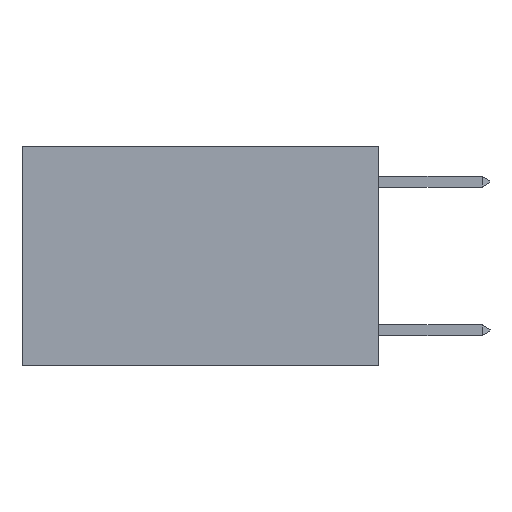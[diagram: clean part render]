
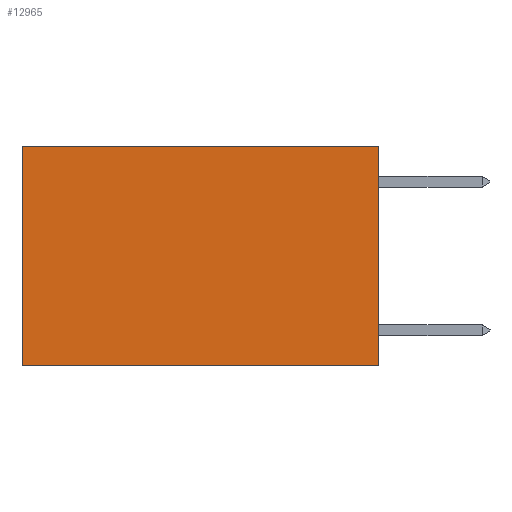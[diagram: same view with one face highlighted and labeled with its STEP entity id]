
A CAD part, left-side view. The second image highlights one B-rep face of the part: STEP entity #12965.
In plain terms, the highlighted planar face has unit normal (-1, 0, 0).
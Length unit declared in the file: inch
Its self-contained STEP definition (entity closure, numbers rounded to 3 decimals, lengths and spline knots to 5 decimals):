
#112 = VERTEX_POINT ( 'NONE', #4835 ) ;
#635 = DIRECTION ( 'NONE',  ( 0., 0., -1. ) ) ;
#2063 = FACE_OUTER_BOUND ( 'NONE', #7457, .T. ) ;
#2075 = EDGE_CURVE ( 'NONE', #17356, #7688, #20302, .T. ) ;
#2147 = EDGE_CURVE ( 'NONE', #112, #8916, #19720, .T. ) ;
#3076 = DIRECTION ( 'NONE',  ( 0., 1., 0. ) ) ;
#3376 = AXIS2_PLACEMENT_3D ( 'NONE', #9734, #11504, #635 ) ;
#4444 = EDGE_CURVE ( 'NONE', #8916, #7688, #9102, .T. ) ;
#4835 = CARTESIAN_POINT ( 'NONE',  ( 0.2625, 0., 0. ) ) ;
#5804 = CARTESIAN_POINT ( 'NONE',  ( 0.2625, 0.6, -0.37 ) ) ;
#7457 = EDGE_LOOP ( 'NONE', ( #9410, #13491, #9125, #22528 ) ) ;
#7688 = VERTEX_POINT ( 'NONE', #5804 ) ;
#8466 = CARTESIAN_POINT ( 'NONE',  ( 0.2625, 0., -0.37 ) ) ;
#8916 = VERTEX_POINT ( 'NONE', #8466 ) ;
#9102 = LINE ( 'NONE', #14715, #9173 ) ;
#9125 = ORIENTED_EDGE ( 'NONE', *, *, #2147, .F. ) ;
#9173 = VECTOR ( 'NONE', #14642, 39.37008 ) ;
#9410 = ORIENTED_EDGE ( 'NONE', *, *, #2075, .T. ) ;
#9734 = CARTESIAN_POINT ( 'NONE',  ( 0.2625, 0., 0. ) ) ;
#10377 = VECTOR ( 'NONE', #3076, 39.37008 ) ;
#10526 = LINE ( 'NONE', #11964, #10377 ) ;
#11433 = EDGE_CURVE ( 'NONE', #112, #17356, #10526, .T. ) ;
#11504 = DIRECTION ( 'NONE',  ( 1., 0., 0. ) ) ;
#11964 = CARTESIAN_POINT ( 'NONE',  ( 0.2625, 0., 0. ) ) ;
#12965 = ADVANCED_FACE ( 'NONE', ( #2063 ), #20091, .F. ) ;
#13491 = ORIENTED_EDGE ( 'NONE', *, *, #4444, .F. ) ;
#14642 = DIRECTION ( 'NONE',  ( 0., 1., 0. ) ) ;
#14715 = CARTESIAN_POINT ( 'NONE',  ( 0.2625, 0., -0.37 ) ) ;
#16271 = CARTESIAN_POINT ( 'NONE',  ( 0.2625, 0.6, 0. ) ) ;
#17356 = VERTEX_POINT ( 'NONE', #16271 ) ;
#18442 = DIRECTION ( 'NONE',  ( 0., 0., -1. ) ) ;
#18527 = CARTESIAN_POINT ( 'NONE',  ( 0.2625, 0., 0. ) ) ;
#19541 = VECTOR ( 'NONE', #18442, 39.37008 ) ;
#19720 = LINE ( 'NONE', #18527, #19541 ) ;
#19734 = DIRECTION ( 'NONE',  ( 0., 0., -1. ) ) ;
#20091 = PLANE ( 'NONE',  #3376 ) ;
#20137 = CARTESIAN_POINT ( 'NONE',  ( 0.2625, 0.6, 0. ) ) ;
#20241 = VECTOR ( 'NONE', #19734, 39.37008 ) ;
#20302 = LINE ( 'NONE', #20137, #20241 ) ;
#22528 = ORIENTED_EDGE ( 'NONE', *, *, #11433, .T. ) ;
